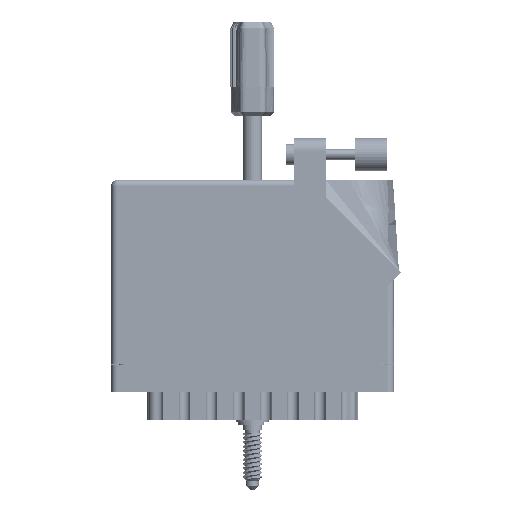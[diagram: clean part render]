
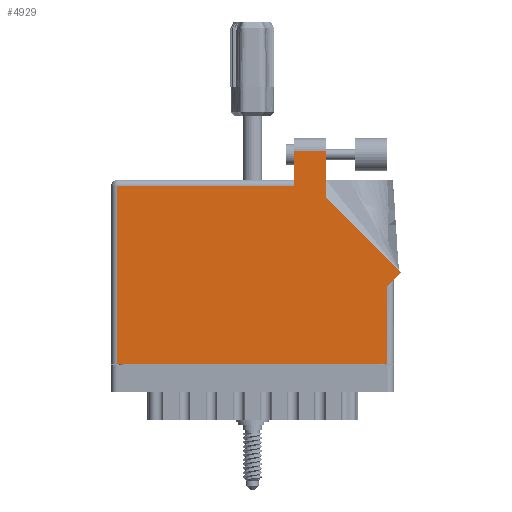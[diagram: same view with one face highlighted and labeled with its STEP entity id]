
A CAD part, front view. The second image highlights one B-rep face of the part: STEP entity #4929.
In plain terms, the highlighted face is planar.
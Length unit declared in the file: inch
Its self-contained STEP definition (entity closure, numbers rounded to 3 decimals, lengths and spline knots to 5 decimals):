
#10 = FACE_OUTER_BOUND ( 'NONE', #8421, .T. ) ;
#3007 = ORIENTED_EDGE ( 'NONE', *, *, #70183, .T. ) ;
#3579 = DIRECTION ( 'NONE',  ( -1., 0., 0. ) ) ;
#4581 = CARTESIAN_POINT ( 'NONE',  ( 2.656, 0.815, 0. ) ) ;
#4738 = CARTESIAN_POINT ( 'NONE',  ( 2.656, 0.753, 0. ) ) ;
#4929 = ADVANCED_FACE ( 'NONE', ( #10 ), #17615, .F. ) ;
#7584 = EDGE_CURVE ( 'NONE', #10176, #30626, #35020, .T. ) ;
#8421 = EDGE_LOOP ( 'NONE', ( #81939, #3007, #85172, #47715, #41331, #46946, #15318, #56984, #68881 ) ) ;
#9347 = CARTESIAN_POINT ( 'NONE',  ( 0., 1.713, 0. ) ) ;
#9786 = VERTEX_POINT ( 'NONE', #21163 ) ;
#10056 = CARTESIAN_POINT ( 'NONE',  ( 0., 0., 0. ) ) ;
#10176 = VERTEX_POINT ( 'NONE', #88350 ) ;
#10217 = CARTESIAN_POINT ( 'NONE',  ( 0.062, 0., 0. ) ) ;
#12167 = DIRECTION ( 'NONE',  ( 0., 1., 0. ) ) ;
#15318 = ORIENTED_EDGE ( 'NONE', *, *, #68475, .T. ) ;
#17018 = EDGE_CURVE ( 'NONE', #9786, #10176, #48246, .T. ) ;
#17022 = EDGE_CURVE ( 'NONE', #76776, #68676, #28922, .T. ) ;
#17615 = PLANE ( 'NONE',  #87301 ) ;
#20173 = EDGE_CURVE ( 'NONE', #60930, #55739, #79046, .T. ) ;
#21163 = CARTESIAN_POINT ( 'NONE',  ( 1.758, 2.05, 0. ) ) ;
#25183 = CARTESIAN_POINT ( 'NONE',  ( 2.78871, 0.88571, 0. ) ) ;
#25903 = DIRECTION ( 'NONE',  ( -0.707, 0.707, 0. ) ) ;
#27042 = VERTEX_POINT ( 'NONE', #25183 ) ;
#28922 = LINE ( 'NONE', #10056, #78421 ) ;
#29280 = VECTOR ( 'NONE', #53317, 39.37008 ) ;
#30040 = CARTESIAN_POINT ( 'NONE',  ( 1.758, 1.775, 0. ) ) ;
#30626 = VERTEX_POINT ( 'NONE', #70601 ) ;
#30637 = DIRECTION ( 'NONE',  ( -1., 0., 0. ) ) ;
#32244 = LINE ( 'NONE', #88615, #42934 ) ;
#33577 = CARTESIAN_POINT ( 'NONE',  ( 2.656, 0., 0. ) ) ;
#35020 = LINE ( 'NONE', #9347, #89064 ) ;
#35413 = VECTOR ( 'NONE', #38387, 39.37008 ) ;
#38387 = DIRECTION ( 'NONE',  ( 0., 1., 0. ) ) ;
#39747 = LINE ( 'NONE', #4581, #35413 ) ;
#39907 = CARTESIAN_POINT ( 'NONE',  ( 2.065, 1.60942, 0. ) ) ;
#41018 = EDGE_CURVE ( 'NONE', #27042, #60930, #32244, .T. ) ;
#41331 = ORIENTED_EDGE ( 'NONE', *, *, #75037, .T. ) ;
#42934 = VECTOR ( 'NONE', #25903, 39.37008 ) ;
#44142 = DIRECTION ( 'NONE',  ( 1., 0., 0. ) ) ;
#45811 = DIRECTION ( 'NONE',  ( 0., -1., 0. ) ) ;
#46946 = ORIENTED_EDGE ( 'NONE', *, *, #17022, .T. ) ;
#47715 = ORIENTED_EDGE ( 'NONE', *, *, #7584, .T. ) ;
#48246 = LINE ( 'NONE', #30040, #62257 ) ;
#50504 = DIRECTION ( 'NONE',  ( 0., -1., 0. ) ) ;
#52395 = EDGE_CURVE ( 'NONE', #60192, #27042, #74454, .T. ) ;
#53218 = VECTOR ( 'NONE', #12167, 39.37008 ) ;
#53317 = DIRECTION ( 'NONE',  ( 0.707, 0.707, 0. ) ) ;
#54115 = CARTESIAN_POINT ( 'NONE',  ( 1.758, 2.05, 0. ) ) ;
#55461 = LINE ( 'NONE', #10217, #88899 ) ;
#55739 = VERTEX_POINT ( 'NONE', #77928 ) ;
#56984 = ORIENTED_EDGE ( 'NONE', *, *, #52395, .T. ) ;
#60192 = VERTEX_POINT ( 'NONE', #4738 ) ;
#60930 = VERTEX_POINT ( 'NONE', #74215 ) ;
#62257 = VECTOR ( 'NONE', #50504, 39.37008 ) ;
#64485 = CARTESIAN_POINT ( 'NONE',  ( 0.062, 0., 0. ) ) ;
#67157 = CARTESIAN_POINT ( 'NONE',  ( 2.718, 0.815, 0. ) ) ;
#68475 = EDGE_CURVE ( 'NONE', #68676, #60192, #39747, .T. ) ;
#68676 = VERTEX_POINT ( 'NONE', #33577 ) ;
#68881 = ORIENTED_EDGE ( 'NONE', *, *, #41018, .T. ) ;
#70183 = EDGE_CURVE ( 'NONE', #55739, #9786, #87076, .T. ) ;
#70601 = CARTESIAN_POINT ( 'NONE',  ( 0.062, 1.713, 0. ) ) ;
#72170 = CARTESIAN_POINT ( 'NONE',  ( 0., 1.775, 0. ) ) ;
#74215 = CARTESIAN_POINT ( 'NONE',  ( 2.065, 1.60942, 0. ) ) ;
#74454 = LINE ( 'NONE', #67157, #29280 ) ;
#75037 = EDGE_CURVE ( 'NONE', #30626, #76776, #55461, .T. ) ;
#76776 = VERTEX_POINT ( 'NONE', #64485 ) ;
#77928 = CARTESIAN_POINT ( 'NONE',  ( 2.065, 2.05, 0. ) ) ;
#78421 = VECTOR ( 'NONE', #44142, 39.37008 ) ;
#79046 = LINE ( 'NONE', #39907, #53218 ) ;
#79696 = DIRECTION ( 'NONE',  ( 0., 0., -1. ) ) ;
#80494 = VECTOR ( 'NONE', #80614, 39.37008 ) ;
#80614 = DIRECTION ( 'NONE',  ( -1., 0., 0. ) ) ;
#81939 = ORIENTED_EDGE ( 'NONE', *, *, #20173, .T. ) ;
#85172 = ORIENTED_EDGE ( 'NONE', *, *, #17018, .T. ) ;
#87076 = LINE ( 'NONE', #54115, #80494 ) ;
#87301 = AXIS2_PLACEMENT_3D ( 'NONE', #72170, #79696, #30637 ) ;
#88350 = CARTESIAN_POINT ( 'NONE',  ( 1.758, 1.713, 0. ) ) ;
#88615 = CARTESIAN_POINT ( 'NONE',  ( 2.78871, 0.88571, 0. ) ) ;
#88899 = VECTOR ( 'NONE', #45811, 39.37008 ) ;
#89064 = VECTOR ( 'NONE', #3579, 39.37008 ) ;
